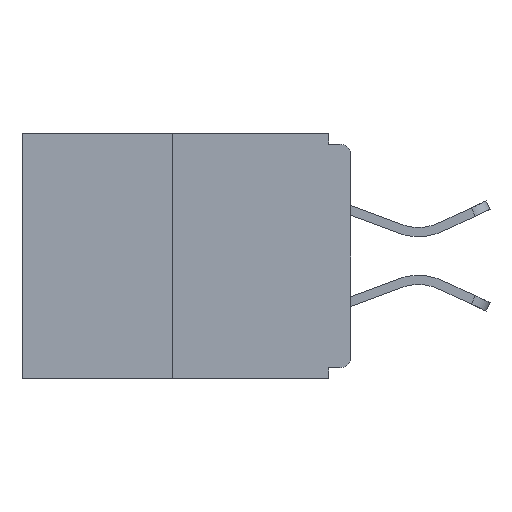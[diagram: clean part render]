
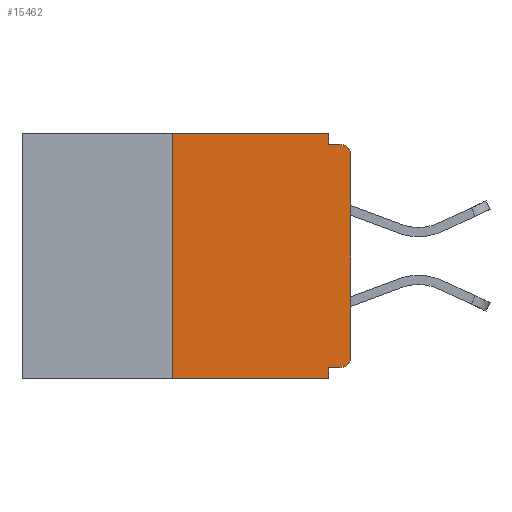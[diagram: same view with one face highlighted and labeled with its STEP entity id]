
A CAD part, left-side view. The second image highlights one B-rep face of the part: STEP entity #15462.
In plain terms, the highlighted planar face has unit normal (-1, 0, 0).
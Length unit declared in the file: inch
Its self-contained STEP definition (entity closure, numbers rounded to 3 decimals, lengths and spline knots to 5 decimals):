
#40 = CARTESIAN_POINT ( 'NONE',  ( 0., 0.46, 0. ) ) ;
#247 = LINE ( 'NONE', #16174, #6485 ) ;
#347 = VERTEX_POINT ( 'NONE', #11579 ) ;
#565 = CARTESIAN_POINT ( 'NONE',  ( 0., 0.25, -0.343 ) ) ;
#888 = CARTESIAN_POINT ( 'NONE',  ( 0., 0.46, -0.343 ) ) ;
#984 = CIRCLE ( 'NONE', #17588, 0.015 ) ;
#1371 = CARTESIAN_POINT ( 'NONE',  ( 0., 0.031, 0. ) ) ;
#1839 = ORIENTED_EDGE ( 'NONE', *, *, #17054, .F. ) ;
#1862 = CARTESIAN_POINT ( 'NONE',  ( 0., 0.031, -0.015 ) ) ;
#1880 = CARTESIAN_POINT ( 'NONE',  ( 0., 0., -0.03 ) ) ;
#2247 = EDGE_CURVE ( 'NONE', #9388, #14089, #9510, .T. ) ;
#2444 = CARTESIAN_POINT ( 'NONE',  ( 0., 0., -0.015 ) ) ;
#2607 = CARTESIAN_POINT ( 'NONE',  ( 0., 0., -0.328 ) ) ;
#2995 = ORIENTED_EDGE ( 'NONE', *, *, #2247, .T. ) ;
#3294 = CARTESIAN_POINT ( 'NONE',  ( 0., 0.031, -0.343 ) ) ;
#3606 = VERTEX_POINT ( 'NONE', #1862 ) ;
#4120 = DIRECTION ( 'NONE',  ( 1., 0., 0. ) ) ;
#4177 = DIRECTION ( 'NONE',  ( -1., 0., 0. ) ) ;
#4273 = ORIENTED_EDGE ( 'NONE', *, *, #17482, .F. ) ;
#4284 = EDGE_LOOP ( 'NONE', ( #19457, #7343, #2995, #10105, #7199, #17764, #16051, #12045, #4273, #1839 ) ) ;
#4748 = CARTESIAN_POINT ( 'NONE',  ( 0., 0.25, 0. ) ) ;
#4865 = CARTESIAN_POINT ( 'NONE',  ( 0., 0., -0.313 ) ) ;
#4877 = VERTEX_POINT ( 'NONE', #5969 ) ;
#5548 = VECTOR ( 'NONE', #8885, 39.37008 ) ;
#5587 = CARTESIAN_POINT ( 'NONE',  ( 0., 0.46, 0. ) ) ;
#5627 = FACE_OUTER_BOUND ( 'NONE', #4284, .T. ) ;
#5969 = CARTESIAN_POINT ( 'NONE',  ( 0., 0.031, -0.328 ) ) ;
#6447 = DIRECTION ( 'NONE',  ( 0., -1., 0. ) ) ;
#6485 = VECTOR ( 'NONE', #14517, 39.37008 ) ;
#6919 = VECTOR ( 'NONE', #13172, 39.37008 ) ;
#7011 = VECTOR ( 'NONE', #15024, 39.37008 ) ;
#7034 = DIRECTION ( 'NONE',  ( 0., 0., -1. ) ) ;
#7199 = ORIENTED_EDGE ( 'NONE', *, *, #7425, .F. ) ;
#7321 = DIRECTION ( 'NONE',  ( 0., 0., -1. ) ) ;
#7343 = ORIENTED_EDGE ( 'NONE', *, *, #10411, .F. ) ;
#7425 = EDGE_CURVE ( 'NONE', #12780, #4877, #18332, .T. ) ;
#8420 = LINE ( 'NONE', #3294, #6919 ) ;
#8677 = PLANE ( 'NONE',  #13516 ) ;
#8874 = VECTOR ( 'NONE', #7321, 39.37008 ) ;
#8885 = DIRECTION ( 'NONE',  ( 0., 1., 0. ) ) ;
#9388 = VERTEX_POINT ( 'NONE', #565 ) ;
#9510 = LINE ( 'NONE', #888, #7011 ) ;
#10105 = ORIENTED_EDGE ( 'NONE', *, *, #14832, .F. ) ;
#10163 = DIRECTION ( 'NONE',  ( 0., 0., 1. ) ) ;
#10411 = EDGE_CURVE ( 'NONE', #9388, #12475, #15436, .T. ) ;
#10450 = DIRECTION ( 'NONE',  ( 0., 0., -1. ) ) ;
#10689 = EDGE_CURVE ( 'NONE', #12780, #18910, #984, .T. ) ;
#11133 = EDGE_CURVE ( 'NONE', #20123, #14787, #13052, .T. ) ;
#11168 = VECTOR ( 'NONE', #10163, 39.37008 ) ;
#11355 = EDGE_CURVE ( 'NONE', #18910, #20123, #247, .T. ) ;
#11579 = CARTESIAN_POINT ( 'NONE',  ( 0., 0.031, 0. ) ) ;
#11887 = LINE ( 'NONE', #1371, #8874 ) ;
#11964 = EDGE_CURVE ( 'NONE', #12475, #347, #19012, .T. ) ;
#12045 = ORIENTED_EDGE ( 'NONE', *, *, #11133, .T. ) ;
#12475 = VERTEX_POINT ( 'NONE', #4748 ) ;
#12780 = VERTEX_POINT ( 'NONE', #19800 ) ;
#13052 = CIRCLE ( 'NONE', #17708, 0.015 ) ;
#13172 = DIRECTION ( 'NONE',  ( 0., 0., -1. ) ) ;
#13425 = DIRECTION ( 'NONE',  ( -1., 0., 0. ) ) ;
#13516 = AXIS2_PLACEMENT_3D ( 'NONE', #5587, #4120, #10450 ) ;
#13675 = DIRECTION ( 'NONE',  ( 0., -1., 0. ) ) ;
#14089 = VERTEX_POINT ( 'NONE', #20496 ) ;
#14517 = DIRECTION ( 'NONE',  ( 0., 0., 1. ) ) ;
#14787 = VERTEX_POINT ( 'NONE', #19233 ) ;
#14832 = EDGE_CURVE ( 'NONE', #4877, #14089, #8420, .T. ) ;
#15024 = DIRECTION ( 'NONE',  ( 0., -1., 0. ) ) ;
#15393 = VECTOR ( 'NONE', #13675, 39.37008 ) ;
#15436 = LINE ( 'NONE', #18340, #11168 ) ;
#15462 = ADVANCED_FACE ( 'NONE', ( #5627 ), #8677, .F. ) ;
#16051 = ORIENTED_EDGE ( 'NONE', *, *, #11355, .T. ) ;
#16174 = CARTESIAN_POINT ( 'NONE',  ( 0., 0., 0. ) ) ;
#16487 = CARTESIAN_POINT ( 'NONE',  ( 0., 0.015, -0.03 ) ) ;
#16713 = DIRECTION ( 'NONE',  ( 0., 0., -1. ) ) ;
#17001 = CARTESIAN_POINT ( 'NONE',  ( 0., 0.015, -0.313 ) ) ;
#17054 = EDGE_CURVE ( 'NONE', #347, #3606, #11887, .T. ) ;
#17482 = EDGE_CURVE ( 'NONE', #3606, #14787, #19123, .T. ) ;
#17588 = AXIS2_PLACEMENT_3D ( 'NONE', #17001, #4177, #16713 ) ;
#17708 = AXIS2_PLACEMENT_3D ( 'NONE', #16487, #13425, #7034 ) ;
#17764 = ORIENTED_EDGE ( 'NONE', *, *, #10689, .T. ) ;
#18332 = LINE ( 'NONE', #2607, #5548 ) ;
#18340 = CARTESIAN_POINT ( 'NONE',  ( 0., 0.25, 0. ) ) ;
#18910 = VERTEX_POINT ( 'NONE', #4865 ) ;
#19012 = LINE ( 'NONE', #40, #19506 ) ;
#19123 = LINE ( 'NONE', #2444, #15393 ) ;
#19233 = CARTESIAN_POINT ( 'NONE',  ( 0., 0.015, -0.015 ) ) ;
#19457 = ORIENTED_EDGE ( 'NONE', *, *, #11964, .F. ) ;
#19506 = VECTOR ( 'NONE', #6447, 39.37008 ) ;
#19800 = CARTESIAN_POINT ( 'NONE',  ( 0., 0.015, -0.328 ) ) ;
#20123 = VERTEX_POINT ( 'NONE', #1880 ) ;
#20496 = CARTESIAN_POINT ( 'NONE',  ( 0., 0.031, -0.343 ) ) ;
